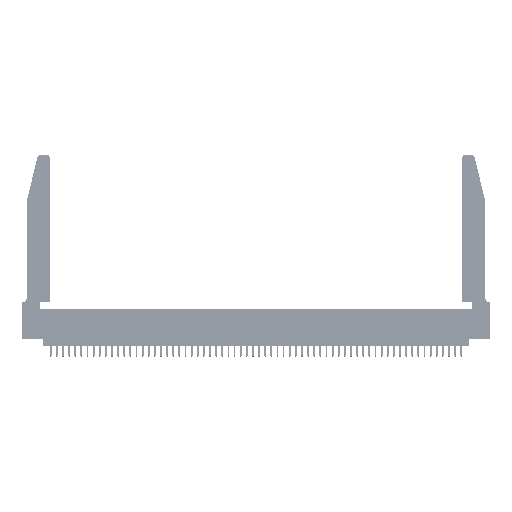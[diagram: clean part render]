
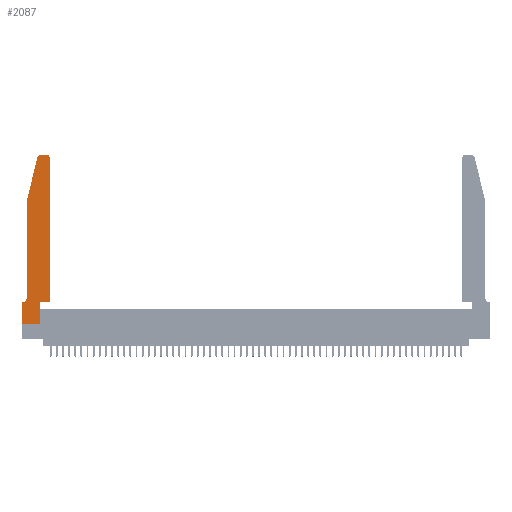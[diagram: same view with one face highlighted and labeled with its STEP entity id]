
A CAD part, top view. The second image highlights one B-rep face of the part: STEP entity #2087.
In plain terms, the highlighted planar face has unit normal (0, 0, 1).
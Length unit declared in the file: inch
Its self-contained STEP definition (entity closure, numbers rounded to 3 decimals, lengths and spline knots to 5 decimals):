
#28 = ORIENTED_EDGE ( 'NONE', *, *, #40109, .T. ) ;
#1435 = CARTESIAN_POINT ( 'NONE',  ( 0.25487, 2.72718, 0.37 ) ) ;
#2087 = ADVANCED_FACE ( 'NONE', ( #7766 ), #38633, .T. ) ;
#2651 = DIRECTION ( 'NONE',  ( -1., 0., 0. ) ) ;
#3205 = LINE ( 'NONE', #21080, #46903 ) ;
#3780 = ORIENTED_EDGE ( 'NONE', *, *, #23795, .T. ) ;
#3898 = ORIENTED_EDGE ( 'NONE', *, *, #39543, .T. ) ;
#4276 = AXIS2_PLACEMENT_3D ( 'NONE', #45032, #40765, #7075 ) ;
#4597 = CARTESIAN_POINT ( 'NONE',  ( 0.4505, 0.35, 0.37 ) ) ;
#5116 = ORIENTED_EDGE ( 'NONE', *, *, #29239, .T. ) ;
#5676 = LINE ( 'NONE', #23922, #16262 ) ;
#7075 = DIRECTION ( 'NONE',  ( -1., 0., 0. ) ) ;
#7433 = VECTOR ( 'NONE', #13883, 39.37008 ) ;
#7766 = FACE_OUTER_BOUND ( 'NONE', #31316, .T. ) ;
#7908 = CARTESIAN_POINT ( 'NONE',  ( 0.2865, 0., 0.37 ) ) ;
#8991 = VECTOR ( 'NONE', #16816, 39.37008 ) ;
#9576 = CARTESIAN_POINT ( 'NONE',  ( 0.0055, 0.35, 0.37 ) ) ;
#10048 = VECTOR ( 'NONE', #29501, 39.37008 ) ;
#10376 = VECTOR ( 'NONE', #42515, 39.37008 ) ;
#11096 = DIRECTION ( 'NONE',  ( 1., 0., 0. ) ) ;
#11895 = LINE ( 'NONE', #24331, #21827 ) ;
#12350 = EDGE_CURVE ( 'NONE', #42101, #44460, #11895, .T. ) ;
#12475 = VECTOR ( 'NONE', #32312, 39.37008 ) ;
#12866 = ORIENTED_EDGE ( 'NONE', *, *, #12350, .T. ) ;
#13883 = DIRECTION ( 'NONE',  ( -0.239, -0.971, 0. ) ) ;
#14421 = CARTESIAN_POINT ( 'NONE',  ( 0., 0., 0.37 ) ) ;
#14548 = EDGE_CURVE ( 'NONE', #20296, #20068, #41450, .T. ) ;
#15550 = CARTESIAN_POINT ( 'NONE',  ( 0., 0.35, 0.37 ) ) ;
#16262 = VECTOR ( 'NONE', #2651, 39.37008 ) ;
#16707 = AXIS2_PLACEMENT_3D ( 'NONE', #51229, #51408, #38792 ) ;
#16816 = DIRECTION ( 'NONE',  ( -1., 0., 0. ) ) ;
#19198 = VERTEX_POINT ( 'NONE', #30184 ) ;
#19770 = VERTEX_POINT ( 'NONE', #7908 ) ;
#20068 = VERTEX_POINT ( 'NONE', #1435 ) ;
#20296 = VERTEX_POINT ( 'NONE', #54364 ) ;
#21080 = CARTESIAN_POINT ( 'NONE',  ( 0.0755, 2., 0.37 ) ) ;
#21267 = DIRECTION ( 'NONE',  ( 0., -1., 0. ) ) ;
#21827 = VECTOR ( 'NONE', #24698, 39.37008 ) ;
#21973 = CARTESIAN_POINT ( 'NONE',  ( 0., 0.35, 0.37 ) ) ;
#22059 = ORIENTED_EDGE ( 'NONE', *, *, #36998, .T. ) ;
#22714 = DIRECTION ( 'NONE',  ( 1., 0., 0. ) ) ;
#23795 = EDGE_CURVE ( 'NONE', #20068, #44491, #37919, .T. ) ;
#23922 = CARTESIAN_POINT ( 'NONE',  ( 0.2605, 2.75, 0.37 ) ) ;
#23995 = LINE ( 'NONE', #25804, #10048 ) ;
#24319 = LINE ( 'NONE', #46418, #10376 ) ;
#24331 = CARTESIAN_POINT ( 'NONE',  ( 0., 0., 0.37 ) ) ;
#24698 = DIRECTION ( 'NONE',  ( 0., -1., 0. ) ) ;
#25130 = CARTESIAN_POINT ( 'NONE',  ( 0.2865, 0.35, 0.37 ) ) ;
#25804 = CARTESIAN_POINT ( 'NONE',  ( 0.2865, 0.35, 0.37 ) ) ;
#26228 = VERTEX_POINT ( 'NONE', #4597 ) ;
#26520 = CARTESIAN_POINT ( 'NONE',  ( 0.0755, 2., 0.37 ) ) ;
#26576 = EDGE_CURVE ( 'NONE', #26228, #39499, #38992, .T. ) ;
#28023 = LINE ( 'NONE', #31881, #45207 ) ;
#28254 = VERTEX_POINT ( 'NONE', #25130 ) ;
#28543 = ORIENTED_EDGE ( 'NONE', *, *, #49233, .T. ) ;
#29239 = EDGE_CURVE ( 'NONE', #54858, #42517, #48660, .T. ) ;
#29244 = CARTESIAN_POINT ( 'NONE',  ( 0.0755, 0.35, 0.37 ) ) ;
#29501 = DIRECTION ( 'NONE',  ( 0., 1., 0. ) ) ;
#29618 = ORIENTED_EDGE ( 'NONE', *, *, #54127, .T. ) ;
#30184 = CARTESIAN_POINT ( 'NONE',  ( 0.4205, 2.75, 0.37 ) ) ;
#30706 = DIRECTION ( 'NONE',  ( 0., 0., 1. ) ) ;
#31316 = EDGE_LOOP ( 'NONE', ( #50317, #36284, #3780, #3898, #5116, #28543, #12866, #28, #22059, #29618, #51307, #46888 ) ) ;
#31881 = CARTESIAN_POINT ( 'NONE',  ( 0.4505, 0.35, 0.37 ) ) ;
#32312 = DIRECTION ( 'NONE',  ( 0., 1., 0. ) ) ;
#35108 = DIRECTION ( 'NONE',  ( 0., 0., 1. ) ) ;
#36284 = ORIENTED_EDGE ( 'NONE', *, *, #14548, .T. ) ;
#36998 = EDGE_CURVE ( 'NONE', #19770, #28254, #23995, .T. ) ;
#37919 = LINE ( 'NONE', #26520, #7433 ) ;
#38633 = PLANE ( 'NONE',  #46052 ) ;
#38792 = DIRECTION ( 'NONE',  ( 1., 0., 0. ) ) ;
#38992 = LINE ( 'NONE', #41007, #12475 ) ;
#39499 = VERTEX_POINT ( 'NONE', #41683 ) ;
#39543 = EDGE_CURVE ( 'NONE', #44491, #54858, #3205, .T. ) ;
#40109 = EDGE_CURVE ( 'NONE', #44460, #19770, #24319, .T. ) ;
#40219 = EDGE_CURVE ( 'NONE', #39499, #19198, #47497, .T. ) ;
#40765 = DIRECTION ( 'NONE',  ( 0., 0., -1. ) ) ;
#41007 = CARTESIAN_POINT ( 'NONE',  ( 0.4505, 0.35, 0.37 ) ) ;
#41450 = CIRCLE ( 'NONE', #47831, 0.03 ) ;
#41683 = CARTESIAN_POINT ( 'NONE',  ( 0.4505, 2.72, 0.37 ) ) ;
#42101 = VERTEX_POINT ( 'NONE', #15550 ) ;
#42515 = DIRECTION ( 'NONE',  ( 1., 0., 0. ) ) ;
#42517 = VERTEX_POINT ( 'NONE', #9576 ) ;
#43078 = DIRECTION ( 'NONE',  ( 1., 0., 0. ) ) ;
#43817 = CARTESIAN_POINT ( 'NONE',  ( 0.284, 2.72, 0.37 ) ) ;
#43915 = EDGE_CURVE ( 'NONE', #19198, #20296, #5676, .T. ) ;
#44460 = VERTEX_POINT ( 'NONE', #14421 ) ;
#44491 = VERTEX_POINT ( 'NONE', #52781 ) ;
#45032 = CARTESIAN_POINT ( 'NONE',  ( 0.0055, 0.42, 0.37 ) ) ;
#45207 = VECTOR ( 'NONE', #11096, 39.37008 ) ;
#46052 = AXIS2_PLACEMENT_3D ( 'NONE', #21973, #35108, #43078 ) ;
#46244 = CARTESIAN_POINT ( 'NONE',  ( 0.0755, 0.42, 0.37 ) ) ;
#46418 = CARTESIAN_POINT ( 'NONE',  ( 0., 0., 0.37 ) ) ;
#46888 = ORIENTED_EDGE ( 'NONE', *, *, #40219, .T. ) ;
#46903 = VECTOR ( 'NONE', #21267, 39.37008 ) ;
#47497 = CIRCLE ( 'NONE', #16707, 0.03 ) ;
#47831 = AXIS2_PLACEMENT_3D ( 'NONE', #43817, #30706, #22714 ) ;
#48660 = CIRCLE ( 'NONE', #4276, 0.07 ) ;
#49233 = EDGE_CURVE ( 'NONE', #42517, #42101, #52787, .T. ) ;
#50317 = ORIENTED_EDGE ( 'NONE', *, *, #43915, .T. ) ;
#51229 = CARTESIAN_POINT ( 'NONE',  ( 0.4205, 2.72, 0.37 ) ) ;
#51307 = ORIENTED_EDGE ( 'NONE', *, *, #26576, .T. ) ;
#51408 = DIRECTION ( 'NONE',  ( 0., 0., 1. ) ) ;
#52781 = CARTESIAN_POINT ( 'NONE',  ( 0.0755, 2., 0.37 ) ) ;
#52787 = LINE ( 'NONE', #29244, #8991 ) ;
#54127 = EDGE_CURVE ( 'NONE', #28254, #26228, #28023, .T. ) ;
#54364 = CARTESIAN_POINT ( 'NONE',  ( 0.284, 2.75, 0.37 ) ) ;
#54858 = VERTEX_POINT ( 'NONE', #46244 ) ;
